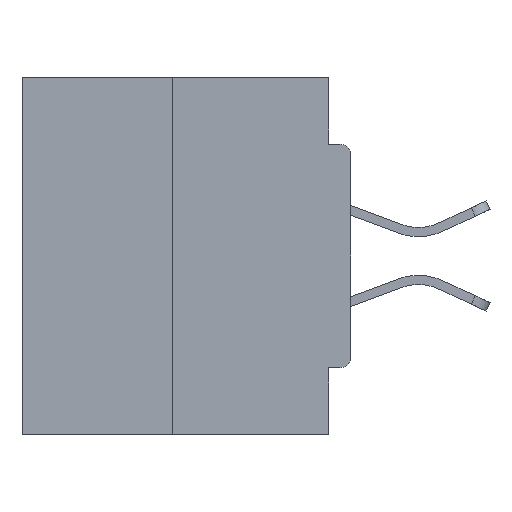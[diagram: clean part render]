
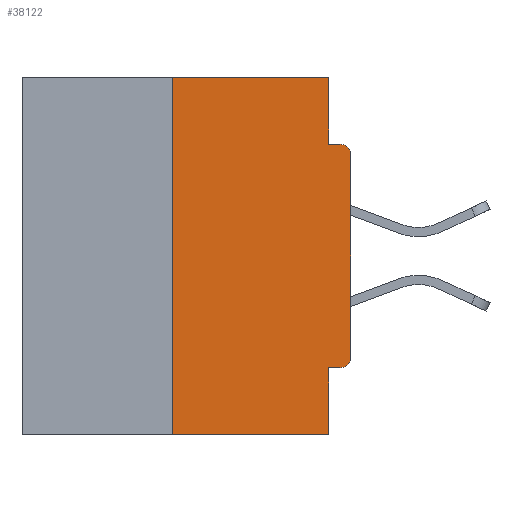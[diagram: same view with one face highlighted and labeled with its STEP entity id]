
A CAD part, left-side view. The second image highlights one B-rep face of the part: STEP entity #38122.
In plain terms, the highlighted planar face has unit normal (-1, 0, 0).
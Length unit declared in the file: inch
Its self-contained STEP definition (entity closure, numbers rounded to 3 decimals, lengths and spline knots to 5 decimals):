
#1449 = VERTEX_POINT ( 'NONE', #14374 ) ;
#3011 = VERTEX_POINT ( 'NONE', #5642 ) ;
#3404 = CARTESIAN_POINT ( 'NONE',  ( 0., 0.25, -0.5 ) ) ;
#3513 = CARTESIAN_POINT ( 'NONE',  ( 0., 0., -0.1085 ) ) ;
#3654 = LINE ( 'NONE', #33045, #5940 ) ;
#3682 = VECTOR ( 'NONE', #6757, 39.37008 ) ;
#3690 = CIRCLE ( 'NONE', #13318, 0.015 ) ;
#4082 = DIRECTION ( 'NONE',  ( 0., 0., -1. ) ) ;
#4634 = EDGE_CURVE ( 'NONE', #12054, #23870, #19824, .T. ) ;
#5332 = PLANE ( 'NONE',  #26358 ) ;
#5398 = CARTESIAN_POINT ( 'NONE',  ( 0., 0.015, -0.0935 ) ) ;
#5527 = CIRCLE ( 'NONE', #19488, 0.015 ) ;
#5642 = CARTESIAN_POINT ( 'NONE',  ( 0., 0., -0.3915 ) ) ;
#5940 = VECTOR ( 'NONE', #30604, 39.37008 ) ;
#6055 = VECTOR ( 'NONE', #27059, 39.37008 ) ;
#6664 = LINE ( 'NONE', #16529, #22364 ) ;
#6692 = CARTESIAN_POINT ( 'NONE',  ( 0., 0.46, 0. ) ) ;
#6757 = DIRECTION ( 'NONE',  ( 0., -1., 0. ) ) ;
#6956 = ORIENTED_EDGE ( 'NONE', *, *, #30078, .F. ) ;
#7191 = CARTESIAN_POINT ( 'NONE',  ( 0., 0.031, -0.5 ) ) ;
#7400 = CARTESIAN_POINT ( 'NONE',  ( 0., 0.015, -0.1085 ) ) ;
#7649 = DIRECTION ( 'NONE',  ( -1., 0., 0. ) ) ;
#7747 = EDGE_CURVE ( 'NONE', #3011, #27129, #12967, .T. ) ;
#7751 = CARTESIAN_POINT ( 'NONE',  ( 0., 0.031, 0. ) ) ;
#8133 = FACE_OUTER_BOUND ( 'NONE', #15548, .T. ) ;
#8493 = EDGE_CURVE ( 'NONE', #27129, #27812, #5527, .T. ) ;
#9799 = EDGE_CURVE ( 'NONE', #36695, #23870, #21596, .T. ) ;
#10988 = LINE ( 'NONE', #6692, #20248 ) ;
#11068 = CARTESIAN_POINT ( 'NONE',  ( 0., 0.46, -0.5 ) ) ;
#11793 = ORIENTED_EDGE ( 'NONE', *, *, #37422, .F. ) ;
#12054 = VERTEX_POINT ( 'NONE', #3404 ) ;
#12597 = DIRECTION ( 'NONE',  ( 0., -1., 0. ) ) ;
#12967 = LINE ( 'NONE', #23944, #6055 ) ;
#13261 = VECTOR ( 'NONE', #38180, 39.37008 ) ;
#13318 = AXIS2_PLACEMENT_3D ( 'NONE', #13722, #28104, #34400 ) ;
#13722 = CARTESIAN_POINT ( 'NONE',  ( 0., 0.015, -0.3915 ) ) ;
#14374 = CARTESIAN_POINT ( 'NONE',  ( 0., 0.25, 0. ) ) ;
#15047 = DIRECTION ( 'NONE',  ( 0., 1., 0. ) ) ;
#15548 = EDGE_LOOP ( 'NONE', ( #25226, #17612, #32206, #18355, #6956, #27211, #27021, #22655, #33608, #11793 ) ) ;
#16285 = EDGE_CURVE ( 'NONE', #17537, #27812, #6664, .T. ) ;
#16529 = CARTESIAN_POINT ( 'NONE',  ( 0., 0., -0.0935 ) ) ;
#17537 = VERTEX_POINT ( 'NONE', #23599 ) ;
#17612 = ORIENTED_EDGE ( 'NONE', *, *, #19626, .F. ) ;
#18355 = ORIENTED_EDGE ( 'NONE', *, *, #9799, .F. ) ;
#19138 = EDGE_CURVE ( 'NONE', #29380, #3011, #3690, .T. ) ;
#19488 = AXIS2_PLACEMENT_3D ( 'NONE', #7400, #7649, #36683 ) ;
#19626 = EDGE_CURVE ( 'NONE', #12054, #1449, #3654, .T. ) ;
#19824 = LINE ( 'NONE', #11068, #3682 ) ;
#20248 = VECTOR ( 'NONE', #12597, 39.37008 ) ;
#21596 = LINE ( 'NONE', #7191, #28073 ) ;
#22043 = LINE ( 'NONE', #7751, #13261 ) ;
#22364 = VECTOR ( 'NONE', #37196, 39.37008 ) ;
#22655 = ORIENTED_EDGE ( 'NONE', *, *, #8493, .T. ) ;
#23589 = LINE ( 'NONE', #28764, #35150 ) ;
#23599 = CARTESIAN_POINT ( 'NONE',  ( 0., 0.031, -0.0935 ) ) ;
#23870 = VERTEX_POINT ( 'NONE', #36208 ) ;
#23944 = CARTESIAN_POINT ( 'NONE',  ( 0., 0., 0. ) ) ;
#25139 = EDGE_CURVE ( 'NONE', #1449, #31275, #10988, .T. ) ;
#25226 = ORIENTED_EDGE ( 'NONE', *, *, #25139, .F. ) ;
#25877 = CARTESIAN_POINT ( 'NONE',  ( 0., 0.46, 0. ) ) ;
#26358 = AXIS2_PLACEMENT_3D ( 'NONE', #25877, #37633, #31955 ) ;
#27021 = ORIENTED_EDGE ( 'NONE', *, *, #7747, .T. ) ;
#27059 = DIRECTION ( 'NONE',  ( 0., 0., 1. ) ) ;
#27129 = VERTEX_POINT ( 'NONE', #3513 ) ;
#27211 = ORIENTED_EDGE ( 'NONE', *, *, #19138, .T. ) ;
#27812 = VERTEX_POINT ( 'NONE', #5398 ) ;
#28073 = VECTOR ( 'NONE', #4082, 39.37008 ) ;
#28104 = DIRECTION ( 'NONE',  ( -1., 0., 0. ) ) ;
#28764 = CARTESIAN_POINT ( 'NONE',  ( 0., 0., -0.4065 ) ) ;
#29380 = VERTEX_POINT ( 'NONE', #31333 ) ;
#30078 = EDGE_CURVE ( 'NONE', #29380, #36695, #23589, .T. ) ;
#30604 = DIRECTION ( 'NONE',  ( 0., 0., 1. ) ) ;
#31275 = VERTEX_POINT ( 'NONE', #34714 ) ;
#31333 = CARTESIAN_POINT ( 'NONE',  ( 0., 0.015, -0.4065 ) ) ;
#31955 = DIRECTION ( 'NONE',  ( 0., 0., -1. ) ) ;
#32206 = ORIENTED_EDGE ( 'NONE', *, *, #4634, .T. ) ;
#33045 = CARTESIAN_POINT ( 'NONE',  ( 0., 0.25, 0. ) ) ;
#33608 = ORIENTED_EDGE ( 'NONE', *, *, #16285, .F. ) ;
#34400 = DIRECTION ( 'NONE',  ( 0., 0., -1. ) ) ;
#34714 = CARTESIAN_POINT ( 'NONE',  ( 0., 0.031, 0. ) ) ;
#35150 = VECTOR ( 'NONE', #15047, 39.37008 ) ;
#36208 = CARTESIAN_POINT ( 'NONE',  ( 0., 0.031, -0.5 ) ) ;
#36668 = CARTESIAN_POINT ( 'NONE',  ( 0., 0.031, -0.4065 ) ) ;
#36683 = DIRECTION ( 'NONE',  ( 0., 0., -1. ) ) ;
#36695 = VERTEX_POINT ( 'NONE', #36668 ) ;
#37196 = DIRECTION ( 'NONE',  ( 0., -1., 0. ) ) ;
#37422 = EDGE_CURVE ( 'NONE', #31275, #17537, #22043, .T. ) ;
#37633 = DIRECTION ( 'NONE',  ( 1., 0., 0. ) ) ;
#38122 = ADVANCED_FACE ( 'NONE', ( #8133 ), #5332, .F. ) ;
#38180 = DIRECTION ( 'NONE',  ( 0., 0., -1. ) ) ;
